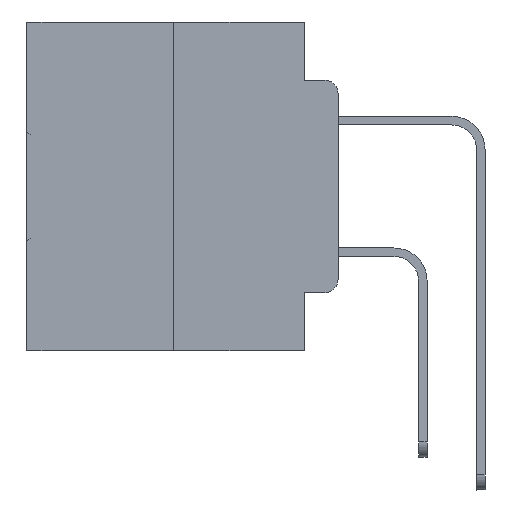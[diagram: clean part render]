
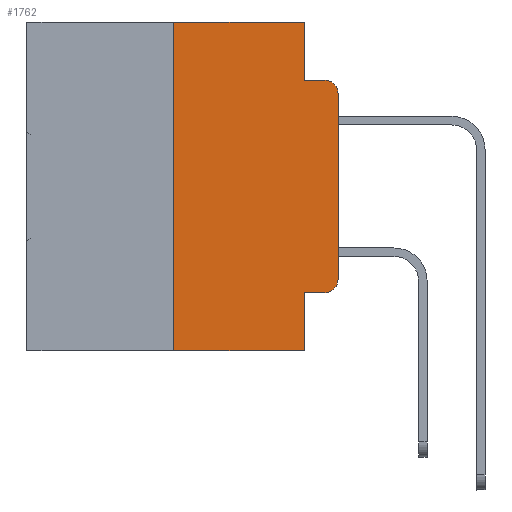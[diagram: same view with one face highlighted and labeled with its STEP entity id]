
A CAD part, left-side view. The second image highlights one B-rep face of the part: STEP entity #1762.
In plain terms, the highlighted planar face has unit normal (-1, 0, 0).
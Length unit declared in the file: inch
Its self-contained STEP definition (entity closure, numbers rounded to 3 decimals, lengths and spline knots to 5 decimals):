
#917 = CIRCLE ( 'NONE', #14173, 0.02 ) ;
#1762 = ADVANCED_FACE ( 'NONE', ( #3530 ), #16559, .F. ) ;
#1978 = VERTEX_POINT ( 'NONE', #14916 ) ;
#2283 = CARTESIAN_POINT ( 'NONE',  ( 0., 0., -0.1085 ) ) ;
#2964 = VERTEX_POINT ( 'NONE', #28882 ) ;
#3084 = CARTESIAN_POINT ( 'NONE',  ( 0., 0.473, -0.5 ) ) ;
#3133 = VECTOR ( 'NONE', #20667, 39.37008 ) ;
#3226 = EDGE_LOOP ( 'NONE', ( #14821, #23036, #27212, #31864, #25405, #17713, #13675, #10878, #22729, #19208 ) ) ;
#3530 = FACE_OUTER_BOUND ( 'NONE', #3226, .T. ) ;
#3886 = VECTOR ( 'NONE', #12075, 39.37008 ) ;
#4718 = EDGE_CURVE ( 'NONE', #14084, #1978, #27706, .T. ) ;
#5645 = VECTOR ( 'NONE', #16174, 39.37008 ) ;
#5718 = VERTEX_POINT ( 'NONE', #2283 ) ;
#6013 = CARTESIAN_POINT ( 'NONE',  ( 0., 0.25, 0. ) ) ;
#6124 = CARTESIAN_POINT ( 'NONE',  ( 0., 0.473, 0. ) ) ;
#6818 = DIRECTION ( 'NONE',  ( 0., -1., 0. ) ) ;
#8800 = CARTESIAN_POINT ( 'NONE',  ( 0., 0.051, 0. ) ) ;
#10092 = LINE ( 'NONE', #11927, #21912 ) ;
#10865 = CARTESIAN_POINT ( 'NONE',  ( 0., 0., 0. ) ) ;
#10878 = ORIENTED_EDGE ( 'NONE', *, *, #32682, .F. ) ;
#11119 = CARTESIAN_POINT ( 'NONE',  ( 0., 0.02, -0.1085 ) ) ;
#11500 = VERTEX_POINT ( 'NONE', #16292 ) ;
#11676 = EDGE_CURVE ( 'NONE', #11500, #29343, #10092, .T. ) ;
#11769 = CARTESIAN_POINT ( 'NONE',  ( 0., 0.25, -0.5 ) ) ;
#11927 = CARTESIAN_POINT ( 'NONE',  ( 0., 0.051, -0.0885 ) ) ;
#12075 = DIRECTION ( 'NONE',  ( 0., -1., 0. ) ) ;
#12440 = LINE ( 'NONE', #6013, #5645 ) ;
#13587 = AXIS2_PLACEMENT_3D ( 'NONE', #28795, #16454, #16519 ) ;
#13675 = ORIENTED_EDGE ( 'NONE', *, *, #16829, .T. ) ;
#13705 = DIRECTION ( 'NONE',  ( 0., 0., -1. ) ) ;
#14084 = VERTEX_POINT ( 'NONE', #31589 ) ;
#14173 = AXIS2_PLACEMENT_3D ( 'NONE', #11119, #28497, #13705 ) ;
#14402 = LINE ( 'NONE', #10865, #27559 ) ;
#14566 = VECTOR ( 'NONE', #28760, 39.37008 ) ;
#14821 = ORIENTED_EDGE ( 'NONE', *, *, #28334, .T. ) ;
#14839 = DIRECTION ( 'NONE',  ( -1., 0., 0. ) ) ;
#14916 = CARTESIAN_POINT ( 'NONE',  ( 0., 0.051, 0. ) ) ;
#15617 = CARTESIAN_POINT ( 'NONE',  ( 0., 0.051, 0. ) ) ;
#16174 = DIRECTION ( 'NONE',  ( 0., 0., 1. ) ) ;
#16255 = VERTEX_POINT ( 'NONE', #23748 ) ;
#16292 = CARTESIAN_POINT ( 'NONE',  ( 0., 0.051, -0.0885 ) ) ;
#16454 = DIRECTION ( 'NONE',  ( 1., 0., 0. ) ) ;
#16519 = DIRECTION ( 'NONE',  ( 0., 0., -1. ) ) ;
#16559 = PLANE ( 'NONE',  #13587 ) ;
#16829 = EDGE_CURVE ( 'NONE', #27919, #16255, #24949, .T. ) ;
#17713 = ORIENTED_EDGE ( 'NONE', *, *, #27121, .F. ) ;
#17862 = EDGE_CURVE ( 'NONE', #2964, #21022, #27542, .T. ) ;
#17955 = CARTESIAN_POINT ( 'NONE',  ( 0., 0.051, -0.4115 ) ) ;
#18111 = LINE ( 'NONE', #8800, #23117 ) ;
#19196 = VECTOR ( 'NONE', #20917, 39.37008 ) ;
#19208 = ORIENTED_EDGE ( 'NONE', *, *, #17862, .T. ) ;
#20168 = EDGE_CURVE ( 'NONE', #5718, #29343, #917, .T. ) ;
#20667 = DIRECTION ( 'NONE',  ( 0., 0., -1. ) ) ;
#20917 = DIRECTION ( 'NONE',  ( 0., -1., 0. ) ) ;
#21022 = VERTEX_POINT ( 'NONE', #32255 ) ;
#21912 = VECTOR ( 'NONE', #6818, 39.37008 ) ;
#22729 = ORIENTED_EDGE ( 'NONE', *, *, #26099, .T. ) ;
#22832 = EDGE_CURVE ( 'NONE', #1978, #11500, #18111, .T. ) ;
#23036 = ORIENTED_EDGE ( 'NONE', *, *, #20168, .T. ) ;
#23117 = VECTOR ( 'NONE', #28723, 39.37008 ) ;
#23279 = LINE ( 'NONE', #26960, #3886 ) ;
#23748 = CARTESIAN_POINT ( 'NONE',  ( 0., 0.051, -0.5 ) ) ;
#24949 = LINE ( 'NONE', #3084, #19196 ) ;
#25405 = ORIENTED_EDGE ( 'NONE', *, *, #4718, .F. ) ;
#26099 = EDGE_CURVE ( 'NONE', #26308, #2964, #23279, .T. ) ;
#26308 = VERTEX_POINT ( 'NONE', #17955 ) ;
#26960 = CARTESIAN_POINT ( 'NONE',  ( 0., 0.051, -0.4115 ) ) ;
#27121 = EDGE_CURVE ( 'NONE', #27919, #14084, #12440, .T. ) ;
#27212 = ORIENTED_EDGE ( 'NONE', *, *, #11676, .F. ) ;
#27542 = CIRCLE ( 'NONE', #29032, 0.02 ) ;
#27559 = VECTOR ( 'NONE', #28249, 39.37008 ) ;
#27706 = LINE ( 'NONE', #6124, #14566 ) ;
#27919 = VERTEX_POINT ( 'NONE', #11769 ) ;
#28249 = DIRECTION ( 'NONE',  ( 0., 0., 1. ) ) ;
#28334 = EDGE_CURVE ( 'NONE', #21022, #5718, #14402, .T. ) ;
#28497 = DIRECTION ( 'NONE',  ( -1., 0., 0. ) ) ;
#28723 = DIRECTION ( 'NONE',  ( 0., 0., -1. ) ) ;
#28760 = DIRECTION ( 'NONE',  ( 0., -1., 0. ) ) ;
#28795 = CARTESIAN_POINT ( 'NONE',  ( 0., 0.473, 0. ) ) ;
#28882 = CARTESIAN_POINT ( 'NONE',  ( 0., 0.02, -0.4115 ) ) ;
#29032 = AXIS2_PLACEMENT_3D ( 'NONE', #29628, #14839, #32105 ) ;
#29091 = LINE ( 'NONE', #15617, #3133 ) ;
#29343 = VERTEX_POINT ( 'NONE', #32094 ) ;
#29628 = CARTESIAN_POINT ( 'NONE',  ( 0., 0.02, -0.3915 ) ) ;
#31589 = CARTESIAN_POINT ( 'NONE',  ( 0., 0.25, 0. ) ) ;
#31864 = ORIENTED_EDGE ( 'NONE', *, *, #22832, .F. ) ;
#32094 = CARTESIAN_POINT ( 'NONE',  ( 0., 0.02, -0.0885 ) ) ;
#32105 = DIRECTION ( 'NONE',  ( 0., 0., -1. ) ) ;
#32255 = CARTESIAN_POINT ( 'NONE',  ( 0., 0., -0.3915 ) ) ;
#32682 = EDGE_CURVE ( 'NONE', #26308, #16255, #29091, .T. ) ;
